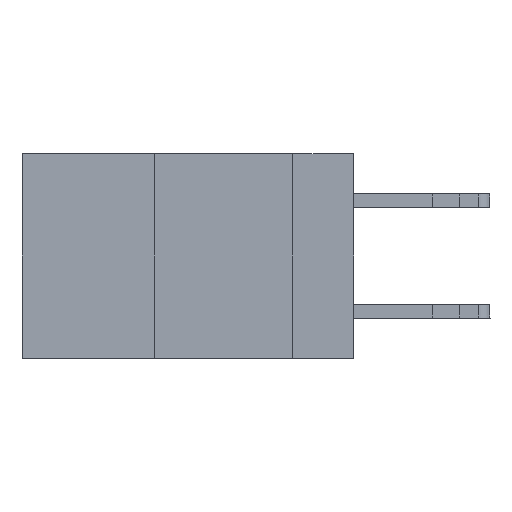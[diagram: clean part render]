
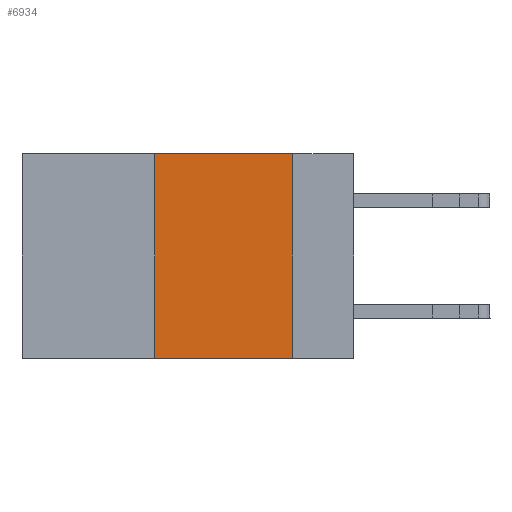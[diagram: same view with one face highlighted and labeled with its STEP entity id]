
A CAD part, left-side view. The second image highlights one B-rep face of the part: STEP entity #6934.
In plain terms, the highlighted planar face has unit normal (-1, 0, 0).
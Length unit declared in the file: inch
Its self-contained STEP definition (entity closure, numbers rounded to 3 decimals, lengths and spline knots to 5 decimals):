
#107 = VERTEX_POINT ( 'NONE', #754 ) ;
#328 = CARTESIAN_POINT ( 'NONE',  ( 0., 0.11, 0. ) ) ;
#754 = CARTESIAN_POINT ( 'NONE',  ( 0., 0.36, -0.37 ) ) ;
#967 = EDGE_CURVE ( 'NONE', #19882, #19737, #5581, .T. ) ;
#1370 = VERTEX_POINT ( 'NONE', #13836 ) ;
#2728 = DIRECTION ( 'NONE',  ( 0., 0., -1. ) ) ;
#2834 = VECTOR ( 'NONE', #9189, 39.37008 ) ;
#3996 = EDGE_LOOP ( 'NONE', ( #14908, #11421, #12827, #9460 ) ) ;
#4239 = DIRECTION ( 'NONE',  ( 1., 0., 0. ) ) ;
#5376 = CARTESIAN_POINT ( 'NONE',  ( 0., 0.6, 0. ) ) ;
#5581 = LINE ( 'NONE', #5376, #14978 ) ;
#6934 = ADVANCED_FACE ( 'NONE', ( #18435 ), #13787, .F. ) ;
#8420 = DIRECTION ( 'NONE',  ( 0., -1., 0. ) ) ;
#9189 = DIRECTION ( 'NONE',  ( 0., 0., 1. ) ) ;
#9336 = DIRECTION ( 'NONE',  ( 0., 0., -1. ) ) ;
#9460 = ORIENTED_EDGE ( 'NONE', *, *, #14572, .T. ) ;
#9599 = EDGE_CURVE ( 'NONE', #19737, #1370, #15539, .T. ) ;
#11421 = ORIENTED_EDGE ( 'NONE', *, *, #967, .F. ) ;
#11994 = AXIS2_PLACEMENT_3D ( 'NONE', #18133, #4239, #2728 ) ;
#12024 = CARTESIAN_POINT ( 'NONE',  ( 0., 0.6, -0.37 ) ) ;
#12827 = ORIENTED_EDGE ( 'NONE', *, *, #12838, .F. ) ;
#12838 = EDGE_CURVE ( 'NONE', #107, #19882, #13867, .T. ) ;
#13787 = PLANE ( 'NONE',  #11994 ) ;
#13836 = CARTESIAN_POINT ( 'NONE',  ( 0., 0.11, -0.37 ) ) ;
#13867 = LINE ( 'NONE', #17332, #2834 ) ;
#13936 = CARTESIAN_POINT ( 'NONE',  ( 0., 0.36, 0. ) ) ;
#14572 = EDGE_CURVE ( 'NONE', #107, #1370, #16589, .T. ) ;
#14585 = CARTESIAN_POINT ( 'NONE',  ( 0., 0.11, 0. ) ) ;
#14908 = ORIENTED_EDGE ( 'NONE', *, *, #9599, .F. ) ;
#14978 = VECTOR ( 'NONE', #8420, 39.37008 ) ;
#15539 = LINE ( 'NONE', #14585, #18093 ) ;
#16589 = LINE ( 'NONE', #12024, #19697 ) ;
#17332 = CARTESIAN_POINT ( 'NONE',  ( 0., 0.36, 0. ) ) ;
#18093 = VECTOR ( 'NONE', #9336, 39.37008 ) ;
#18133 = CARTESIAN_POINT ( 'NONE',  ( 0., 0.6, 0. ) ) ;
#18397 = DIRECTION ( 'NONE',  ( 0., -1., 0. ) ) ;
#18435 = FACE_OUTER_BOUND ( 'NONE', #3996, .T. ) ;
#19697 = VECTOR ( 'NONE', #18397, 39.37008 ) ;
#19737 = VERTEX_POINT ( 'NONE', #328 ) ;
#19882 = VERTEX_POINT ( 'NONE', #13936 ) ;
